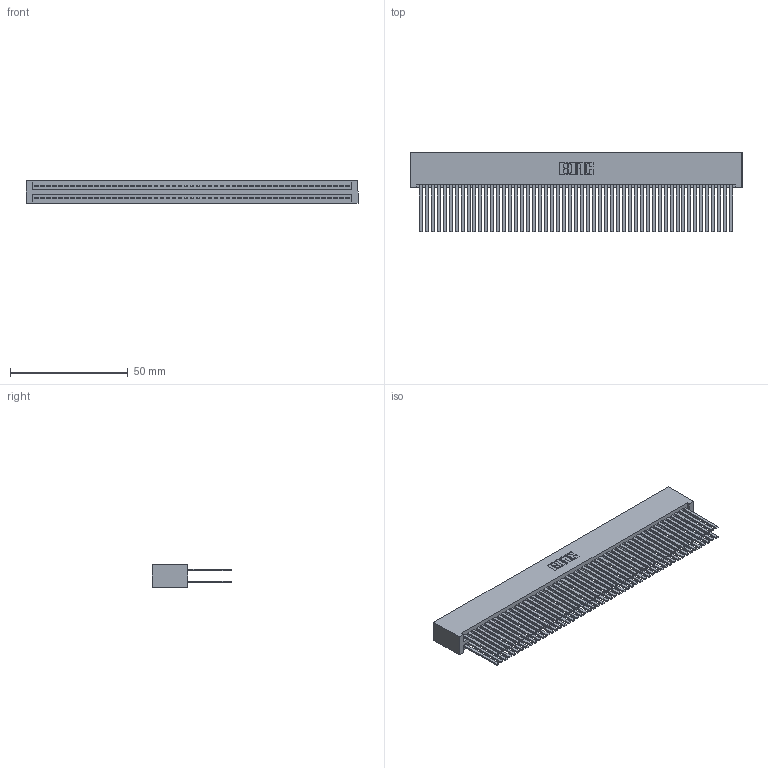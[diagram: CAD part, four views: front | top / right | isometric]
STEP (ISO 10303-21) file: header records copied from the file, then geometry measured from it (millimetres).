
FILE_DESCRIPTION (( 'STEP AP203' ), '1' );
FILE_NAME ('395-106-544-201.STEP', '2019-10-27T05:34:46', ( '' ), ( '' ), 'SwSTEP 2.0', 'SolidWorks 2016', '' );
FILE_SCHEMA (( 'CONFIG_CONTROL_DESIGN' ));
Length unit declared in the file: inch
Products named in the file (3): 395-106-544-201; 345 Part_No Mounting Lugs; 345-292-001_345-293-144
Assembly tree (107 placements, depth 2):
  395-106-544-201
    345 Part_No Mounting Lugs
    345-292-001_345-293-144  x106
Bounding box: 141.22 x 33.96 x 9.4 mm (x, y, z)
Volume: 15922.6 mm3; surface area: 28407.7 mm2
Topology: 107 solids, 107 shells, 4782 faces, 14203 edges, 9326 vertices
Faces by surface type: plane 3150, cylinder 1632
Entity records: 39643 total; most frequent: CARTESIAN_POINT 6632, ORIENTED_EDGE 6566, DIRECTION 5827, EDGE_CURVE 3283, LINE 2951, VECTOR 2951, VERTEX_POINT 2186, AXIS2_PLACEMENT_3D 1438
